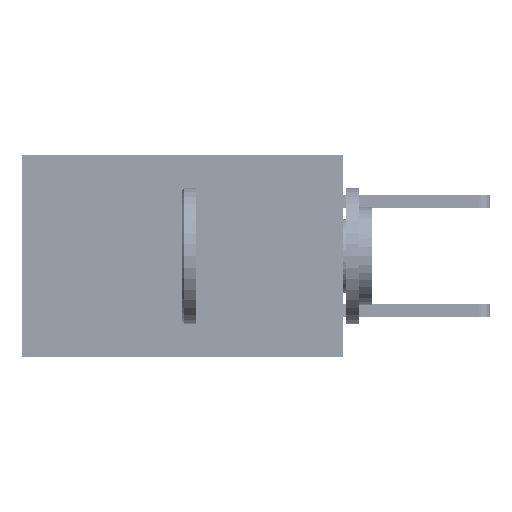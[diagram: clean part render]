
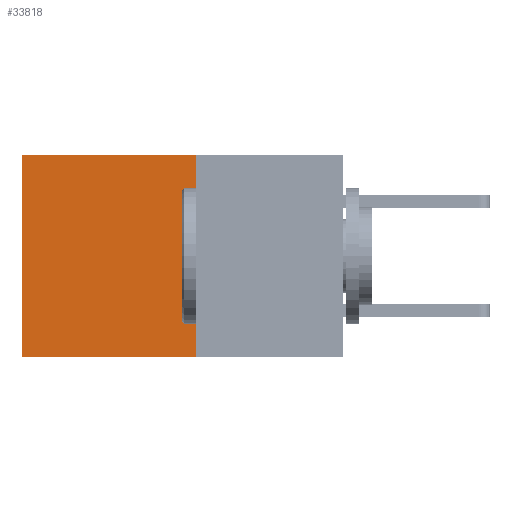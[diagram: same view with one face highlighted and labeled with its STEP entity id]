
A CAD part, left-side view. The second image highlights one B-rep face of the part: STEP entity #33818.
In plain terms, the highlighted planar face has unit normal (-1, 0, 0).
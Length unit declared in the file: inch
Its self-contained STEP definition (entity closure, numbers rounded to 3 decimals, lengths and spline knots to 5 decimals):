
#170 = DIRECTION ( 'NONE',  ( 0., 0., -1. ) ) ;
#869 = PLANE ( 'NONE',  #5176 ) ;
#1402 = VERTEX_POINT ( 'NONE', #18439 ) ;
#1830 = LINE ( 'NONE', #28571, #13967 ) ;
#2792 = ORIENTED_EDGE ( 'NONE', *, *, #14965, .T. ) ;
#3249 = DIRECTION ( 'NONE',  ( 0., 0., -1. ) ) ;
#5176 = AXIS2_PLACEMENT_3D ( 'NONE', #16667, #33041, #170 ) ;
#5954 = FACE_OUTER_BOUND ( 'NONE', #12547, .T. ) ;
#9238 = LINE ( 'NONE', #19963, #14014 ) ;
#9396 = ORIENTED_EDGE ( 'NONE', *, *, #30699, .F. ) ;
#9740 = DIRECTION ( 'NONE',  ( 0., 1., 0. ) ) ;
#11241 = ORIENTED_EDGE ( 'NONE', *, *, #18227, .F. ) ;
#11754 = VECTOR ( 'NONE', #19538, 39.37008 ) ;
#12474 = CARTESIAN_POINT ( 'NONE',  ( 0.277, 0.27, 0. ) ) ;
#12547 = EDGE_LOOP ( 'NONE', ( #2792, #11241, #9396, #29624 ) ) ;
#13092 = CARTESIAN_POINT ( 'NONE',  ( 0.277, 0.27, 0. ) ) ;
#13205 = VERTEX_POINT ( 'NONE', #20726 ) ;
#13967 = VECTOR ( 'NONE', #9740, 39.37008 ) ;
#14014 = VECTOR ( 'NONE', #3249, 39.37008 ) ;
#14965 = EDGE_CURVE ( 'NONE', #31272, #1402, #9238, .T. ) ;
#16502 = EDGE_CURVE ( 'NONE', #20347, #31272, #16880, .T. ) ;
#16667 = CARTESIAN_POINT ( 'NONE',  ( 0.277, 0.27, -0.37 ) ) ;
#16880 = LINE ( 'NONE', #13092, #11754 ) ;
#18227 = EDGE_CURVE ( 'NONE', #13205, #1402, #1830, .T. ) ;
#18439 = CARTESIAN_POINT ( 'NONE',  ( 0.277, 0.59, -0.37 ) ) ;
#19538 = DIRECTION ( 'NONE',  ( 0., 1., 0. ) ) ;
#19963 = CARTESIAN_POINT ( 'NONE',  ( 0.277, 0.59, -0.37 ) ) ;
#20347 = VERTEX_POINT ( 'NONE', #12474 ) ;
#20726 = CARTESIAN_POINT ( 'NONE',  ( 0.277, 0.27, -0.37 ) ) ;
#23997 = LINE ( 'NONE', #28601, #28855 ) ;
#24291 = CARTESIAN_POINT ( 'NONE',  ( 0.277, 0.59, 0. ) ) ;
#28571 = CARTESIAN_POINT ( 'NONE',  ( 0.277, 0.27, -0.37 ) ) ;
#28601 = CARTESIAN_POINT ( 'NONE',  ( 0.277, 0.27, -0.37 ) ) ;
#28855 = VECTOR ( 'NONE', #31724, 39.37008 ) ;
#29624 = ORIENTED_EDGE ( 'NONE', *, *, #16502, .T. ) ;
#30699 = EDGE_CURVE ( 'NONE', #20347, #13205, #23997, .T. ) ;
#31272 = VERTEX_POINT ( 'NONE', #24291 ) ;
#31724 = DIRECTION ( 'NONE',  ( 0., 0., -1. ) ) ;
#33041 = DIRECTION ( 'NONE',  ( 1., 0., 0. ) ) ;
#33818 = ADVANCED_FACE ( 'NONE', ( #5954 ), #869, .F. ) ;
